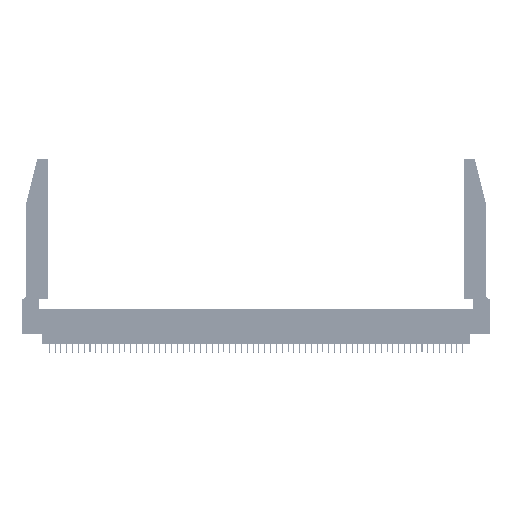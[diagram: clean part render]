
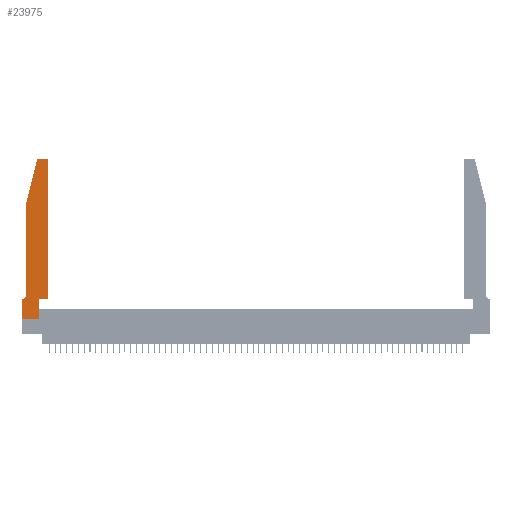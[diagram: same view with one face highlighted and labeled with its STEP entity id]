
A CAD part, top view. The second image highlights one B-rep face of the part: STEP entity #23975.
In plain terms, the highlighted planar face has unit normal (0, 0, 1).
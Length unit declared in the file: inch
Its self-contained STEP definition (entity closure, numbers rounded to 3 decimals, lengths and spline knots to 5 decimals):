
#218 = CARTESIAN_POINT ( 'NONE',  ( 0., 0.35, 0.37 ) ) ;
#1097 = ORIENTED_EDGE ( 'NONE', *, *, #16134, .T. ) ;
#1174 = DIRECTION ( 'NONE',  ( 0., 0., 1. ) ) ;
#1762 = EDGE_CURVE ( 'NONE', #12484, #37530, #32355, .T. ) ;
#3151 = VERTEX_POINT ( 'NONE', #18803 ) ;
#3594 = EDGE_CURVE ( 'NONE', #41022, #3151, #55619, .T. ) ;
#5363 = CARTESIAN_POINT ( 'NONE',  ( 0.2865, 0., 0.37 ) ) ;
#5424 = AXIS2_PLACEMENT_3D ( 'NONE', #218, #31316, #35017 ) ;
#6337 = VERTEX_POINT ( 'NONE', #26131 ) ;
#6698 = VECTOR ( 'NONE', #57362, 39.37008 ) ;
#7014 = AXIS2_PLACEMENT_3D ( 'NONE', #41193, #14626, #40435 ) ;
#7632 = ORIENTED_EDGE ( 'NONE', *, *, #19498, .T. ) ;
#8620 = VERTEX_POINT ( 'NONE', #9270 ) ;
#8723 = VERTEX_POINT ( 'NONE', #5363 ) ;
#9270 = CARTESIAN_POINT ( 'NONE',  ( 0.4505, 0.35, 0.37 ) ) ;
#9431 = CIRCLE ( 'NONE', #14072, 0.03 ) ;
#10000 = DIRECTION ( 'NONE',  ( -1., 0., 0. ) ) ;
#10324 = LINE ( 'NONE', #50586, #35979 ) ;
#10441 = DIRECTION ( 'NONE',  ( 0., 0., 1. ) ) ;
#11158 = DIRECTION ( 'NONE',  ( 0., 1., 0. ) ) ;
#12449 = CARTESIAN_POINT ( 'NONE',  ( 0.0755, 2., 0.37 ) ) ;
#12484 = VERTEX_POINT ( 'NONE', #23717 ) ;
#12582 = EDGE_CURVE ( 'NONE', #8620, #30229, #10324, .T. ) ;
#12607 = CARTESIAN_POINT ( 'NONE',  ( 0.0755, 2., 0.37 ) ) ;
#14072 = AXIS2_PLACEMENT_3D ( 'NONE', #37218, #10441, #28517 ) ;
#14293 = VECTOR ( 'NONE', #54611, 39.37008 ) ;
#14626 = DIRECTION ( 'NONE',  ( 0., 0., -1. ) ) ;
#14697 = LINE ( 'NONE', #12449, #55370 ) ;
#15693 = CARTESIAN_POINT ( 'NONE',  ( 0.0755, 0.42, 0.37 ) ) ;
#16134 = EDGE_CURVE ( 'NONE', #44473, #6337, #17339, .T. ) ;
#16451 = LINE ( 'NONE', #34755, #6698 ) ;
#17339 = CIRCLE ( 'NONE', #7014, 0.07 ) ;
#17558 = ORIENTED_EDGE ( 'NONE', *, *, #54906, .T. ) ;
#18803 = CARTESIAN_POINT ( 'NONE',  ( 0.0755, 2., 0.37 ) ) ;
#19041 = ORIENTED_EDGE ( 'NONE', *, *, #47489, .T. ) ;
#19498 = EDGE_CURVE ( 'NONE', #37530, #41022, #26011, .T. ) ;
#22386 = CARTESIAN_POINT ( 'NONE',  ( 0., 0.35, 0.37 ) ) ;
#23565 = DIRECTION ( 'NONE',  ( 1., 0., 0. ) ) ;
#23573 = CARTESIAN_POINT ( 'NONE',  ( 0., 0., 0.37 ) ) ;
#23717 = CARTESIAN_POINT ( 'NONE',  ( 0.4205, 2.75, 0.37 ) ) ;
#23975 = ADVANCED_FACE ( 'NONE', ( #37696 ), #48939, .T. ) ;
#24705 = VECTOR ( 'NONE', #26693, 39.37008 ) ;
#26011 = CIRCLE ( 'NONE', #37989, 0.03 ) ;
#26131 = CARTESIAN_POINT ( 'NONE',  ( 0.0055, 0.35, 0.37 ) ) ;
#26693 = DIRECTION ( 'NONE',  ( 1., 0., 0. ) ) ;
#26715 = CARTESIAN_POINT ( 'NONE',  ( 0., 0., 0.37 ) ) ;
#27314 = ORIENTED_EDGE ( 'NONE', *, *, #51374, .T. ) ;
#27806 = CARTESIAN_POINT ( 'NONE',  ( 0.284, 2.72, 0.37 ) ) ;
#28209 = EDGE_LOOP ( 'NONE', ( #42541, #7632, #42375, #19041, #1097, #51125, #27314, #56965, #30642, #17558, #45835, #40465 ) ) ;
#28363 = CARTESIAN_POINT ( 'NONE',  ( 0.2865, 0.35, 0.37 ) ) ;
#28517 = DIRECTION ( 'NONE',  ( 1., 0., 0. ) ) ;
#28729 = DIRECTION ( 'NONE',  ( 0., 1., 0. ) ) ;
#28937 = VECTOR ( 'NONE', #10000, 39.37008 ) ;
#30229 = VERTEX_POINT ( 'NONE', #57300 ) ;
#30642 = ORIENTED_EDGE ( 'NONE', *, *, #46737, .T. ) ;
#31316 = DIRECTION ( 'NONE',  ( 0., 0., 1. ) ) ;
#31441 = DIRECTION ( 'NONE',  ( 0., -1., 0. ) ) ;
#32355 = LINE ( 'NONE', #53393, #28937 ) ;
#34755 = CARTESIAN_POINT ( 'NONE',  ( 0.0755, 0.35, 0.37 ) ) ;
#35017 = DIRECTION ( 'NONE',  ( 1., 0., 0. ) ) ;
#35389 = CARTESIAN_POINT ( 'NONE',  ( 0., 0., 0.37 ) ) ;
#35979 = VECTOR ( 'NONE', #28729, 39.37008 ) ;
#36246 = VECTOR ( 'NONE', #52879, 39.37008 ) ;
#36694 = EDGE_CURVE ( 'NONE', #40630, #8723, #54870, .T. ) ;
#37218 = CARTESIAN_POINT ( 'NONE',  ( 0.4205, 2.72, 0.37 ) ) ;
#37530 = VERTEX_POINT ( 'NONE', #41947 ) ;
#37696 = FACE_OUTER_BOUND ( 'NONE', #28209, .T. ) ;
#37746 = CARTESIAN_POINT ( 'NONE',  ( 0.2865, 0.35, 0.37 ) ) ;
#37757 = VECTOR ( 'NONE', #11158, 39.37008 ) ;
#37989 = AXIS2_PLACEMENT_3D ( 'NONE', #27806, #1174, #23565 ) ;
#39659 = DIRECTION ( 'NONE',  ( 1., 0., 0. ) ) ;
#40435 = DIRECTION ( 'NONE',  ( -1., 0., 0. ) ) ;
#40465 = ORIENTED_EDGE ( 'NONE', *, *, #51023, .T. ) ;
#40630 = VERTEX_POINT ( 'NONE', #23573 ) ;
#40676 = LINE ( 'NONE', #26715, #14293 ) ;
#41022 = VERTEX_POINT ( 'NONE', #47889 ) ;
#41193 = CARTESIAN_POINT ( 'NONE',  ( 0.0055, 0.42, 0.37 ) ) ;
#41947 = CARTESIAN_POINT ( 'NONE',  ( 0.284, 2.75, 0.37 ) ) ;
#42375 = ORIENTED_EDGE ( 'NONE', *, *, #3594, .T. ) ;
#42396 = VERTEX_POINT ( 'NONE', #22386 ) ;
#42541 = ORIENTED_EDGE ( 'NONE', *, *, #1762, .T. ) ;
#44145 = EDGE_CURVE ( 'NONE', #6337, #42396, #16451, .T. ) ;
#44278 = VERTEX_POINT ( 'NONE', #28363 ) ;
#44473 = VERTEX_POINT ( 'NONE', #15693 ) ;
#45835 = ORIENTED_EDGE ( 'NONE', *, *, #12582, .T. ) ;
#46737 = EDGE_CURVE ( 'NONE', #8723, #44278, #50201, .T. ) ;
#47489 = EDGE_CURVE ( 'NONE', #3151, #44473, #14697, .T. ) ;
#47889 = CARTESIAN_POINT ( 'NONE',  ( 0.25487, 2.72718, 0.37 ) ) ;
#48249 = LINE ( 'NONE', #52793, #24705 ) ;
#48939 = PLANE ( 'NONE',  #5424 ) ;
#50201 = LINE ( 'NONE', #37746, #37757 ) ;
#50586 = CARTESIAN_POINT ( 'NONE',  ( 0.4505, 0.35, 0.37 ) ) ;
#51023 = EDGE_CURVE ( 'NONE', #30229, #12484, #9431, .T. ) ;
#51125 = ORIENTED_EDGE ( 'NONE', *, *, #44145, .T. ) ;
#51374 = EDGE_CURVE ( 'NONE', #42396, #40630, #40676, .T. ) ;
#52793 = CARTESIAN_POINT ( 'NONE',  ( 0.4505, 0.35, 0.37 ) ) ;
#52879 = DIRECTION ( 'NONE',  ( -0.239, -0.971, 0. ) ) ;
#53393 = CARTESIAN_POINT ( 'NONE',  ( 0.2605, 2.75, 0.37 ) ) ;
#54611 = DIRECTION ( 'NONE',  ( 0., -1., 0. ) ) ;
#54870 = LINE ( 'NONE', #35389, #56248 ) ;
#54906 = EDGE_CURVE ( 'NONE', #44278, #8620, #48249, .T. ) ;
#55370 = VECTOR ( 'NONE', #31441, 39.37008 ) ;
#55619 = LINE ( 'NONE', #12607, #36246 ) ;
#56248 = VECTOR ( 'NONE', #39659, 39.37008 ) ;
#56965 = ORIENTED_EDGE ( 'NONE', *, *, #36694, .T. ) ;
#57300 = CARTESIAN_POINT ( 'NONE',  ( 0.4505, 2.72, 0.37 ) ) ;
#57362 = DIRECTION ( 'NONE',  ( -1., 0., 0. ) ) ;
